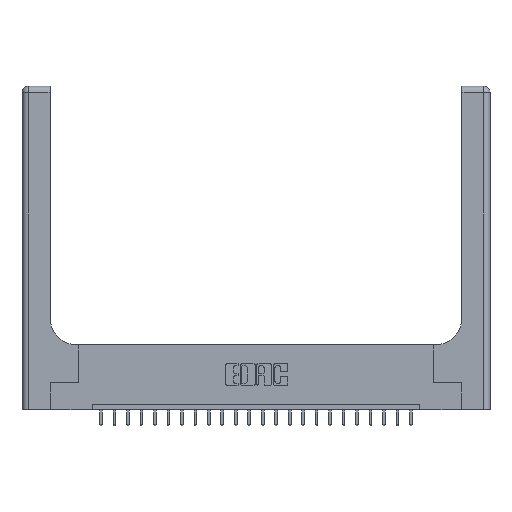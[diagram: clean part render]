
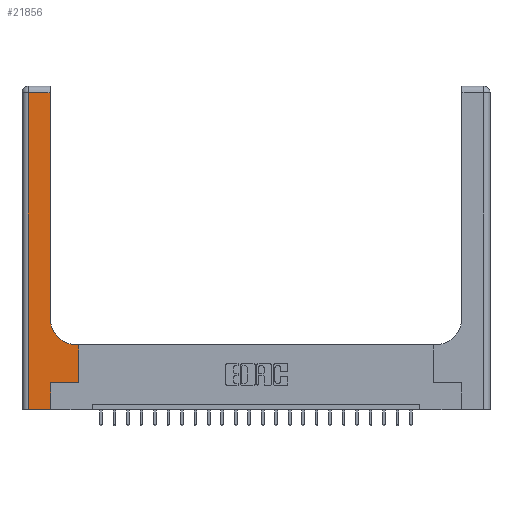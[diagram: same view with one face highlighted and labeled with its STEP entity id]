
A CAD part, top view. The second image highlights one B-rep face of the part: STEP entity #21856.
In plain terms, the highlighted planar face has unit normal (0, 0, 1).
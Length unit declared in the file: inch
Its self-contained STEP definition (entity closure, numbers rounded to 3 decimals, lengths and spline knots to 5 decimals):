
#232 = CARTESIAN_POINT ( 'NONE',  ( 0.265, 0.25, 0.37 ) ) ;
#1228 = CARTESIAN_POINT ( 'NONE',  ( 0.51, 0.6, 0.37 ) ) ;
#2026 = CARTESIAN_POINT ( 'NONE',  ( 0.265, 0., 0.37 ) ) ;
#2142 = DIRECTION ( 'NONE',  ( -1., 0., 0. ) ) ;
#2154 = DIRECTION ( 'NONE',  ( 1., 0., 0. ) ) ;
#2218 = CARTESIAN_POINT ( 'NONE',  ( 0.06, 2.94, 0.37 ) ) ;
#2223 = CARTESIAN_POINT ( 'NONE',  ( 0., 0., 0.37 ) ) ;
#2245 = PLANE ( 'NONE',  #7970 ) ;
#2419 = CARTESIAN_POINT ( 'NONE',  ( 0.528, 0.25, 0.37 ) ) ;
#2725 = DIRECTION ( 'NONE',  ( -1., 0., 0. ) ) ;
#2864 = VERTEX_POINT ( 'NONE', #14669 ) ;
#3715 = CARTESIAN_POINT ( 'NONE',  ( 0.06, 0., 0.37 ) ) ;
#4055 = CARTESIAN_POINT ( 'NONE',  ( 0., 2.94, 0.37 ) ) ;
#4107 = DIRECTION ( 'NONE',  ( 0., 0., -1. ) ) ;
#4255 = VECTOR ( 'NONE', #16063, 39.37008 ) ;
#4325 = DIRECTION ( 'NONE',  ( 0., 0., -1. ) ) ;
#4984 = ORIENTED_EDGE ( 'NONE', *, *, #13553, .T. ) ;
#5240 = VECTOR ( 'NONE', #17815, 39.37008 ) ;
#6204 = LINE ( 'NONE', #20498, #13861 ) ;
#6230 = EDGE_LOOP ( 'NONE', ( #4984, #18419, #7827, #17557, #17902, #16923, #7605, #18739, #9390 ) ) ;
#6245 = LINE ( 'NONE', #2419, #9739 ) ;
#7581 = FACE_OUTER_BOUND ( 'NONE', #6230, .T. ) ;
#7605 = ORIENTED_EDGE ( 'NONE', *, *, #14408, .T. ) ;
#7763 = DIRECTION ( 'NONE',  ( -1., 0., 0. ) ) ;
#7827 = ORIENTED_EDGE ( 'NONE', *, *, #8521, .T. ) ;
#7970 = AXIS2_PLACEMENT_3D ( 'NONE', #19796, #4325, #2142 ) ;
#7999 = LINE ( 'NONE', #4055, #13458 ) ;
#8104 = DIRECTION ( 'NONE',  ( 0., 1., 0. ) ) ;
#8521 = EDGE_CURVE ( 'NONE', #12665, #9909, #20924, .T. ) ;
#8888 = VERTEX_POINT ( 'NONE', #20872 ) ;
#8959 = CARTESIAN_POINT ( 'NONE',  ( 0.26, 0.85, 0.37 ) ) ;
#8989 = LINE ( 'NONE', #2026, #4255 ) ;
#9312 = VECTOR ( 'NONE', #18268, 39.37008 ) ;
#9390 = ORIENTED_EDGE ( 'NONE', *, *, #18151, .T. ) ;
#9608 = VERTEX_POINT ( 'NONE', #11747 ) ;
#9717 = VECTOR ( 'NONE', #21618, 39.37008 ) ;
#9739 = VECTOR ( 'NONE', #8104, 39.37008 ) ;
#9909 = VERTEX_POINT ( 'NONE', #3715 ) ;
#10444 = AXIS2_PLACEMENT_3D ( 'NONE', #21772, #4107, #2154 ) ;
#10702 = VECTOR ( 'NONE', #14161, 39.37008 ) ;
#11173 = LINE ( 'NONE', #18052, #9312 ) ;
#11747 = CARTESIAN_POINT ( 'NONE',  ( 0.528, 0.25, 0.37 ) ) ;
#12427 = CARTESIAN_POINT ( 'NONE',  ( 0.06, 3., 0.37 ) ) ;
#12665 = VERTEX_POINT ( 'NONE', #2218 ) ;
#12693 = CARTESIAN_POINT ( 'NONE',  ( 0.26, 3., 0.37 ) ) ;
#13458 = VECTOR ( 'NONE', #7763, 39.37008 ) ;
#13553 = EDGE_CURVE ( 'NONE', #13951, #2864, #19564, .T. ) ;
#13580 = EDGE_CURVE ( 'NONE', #14258, #9608, #11173, .T. ) ;
#13861 = VECTOR ( 'NONE', #2725, 39.37008 ) ;
#13922 = EDGE_CURVE ( 'NONE', #9909, #8888, #14291, .T. ) ;
#13951 = VERTEX_POINT ( 'NONE', #8959 ) ;
#14161 = DIRECTION ( 'NONE',  ( 0., -1., 0. ) ) ;
#14258 = VERTEX_POINT ( 'NONE', #232 ) ;
#14291 = LINE ( 'NONE', #2223, #9717 ) ;
#14408 = EDGE_CURVE ( 'NONE', #9608, #15280, #6245, .T. ) ;
#14669 = CARTESIAN_POINT ( 'NONE',  ( 0.26, 2.94, 0.37 ) ) ;
#15280 = VERTEX_POINT ( 'NONE', #17758 ) ;
#16063 = DIRECTION ( 'NONE',  ( 0., 1., 0. ) ) ;
#16923 = ORIENTED_EDGE ( 'NONE', *, *, #13580, .T. ) ;
#17557 = ORIENTED_EDGE ( 'NONE', *, *, #13922, .T. ) ;
#17758 = CARTESIAN_POINT ( 'NONE',  ( 0.528, 0.6, 0.37 ) ) ;
#17815 = DIRECTION ( 'NONE',  ( 0., 1., 0. ) ) ;
#17902 = ORIENTED_EDGE ( 'NONE', *, *, #21754, .T. ) ;
#18052 = CARTESIAN_POINT ( 'NONE',  ( 0.265, 0.25, 0.37 ) ) ;
#18151 = EDGE_CURVE ( 'NONE', #21519, #13951, #22324, .T. ) ;
#18268 = DIRECTION ( 'NONE',  ( 1., 0., 0. ) ) ;
#18419 = ORIENTED_EDGE ( 'NONE', *, *, #19125, .T. ) ;
#18739 = ORIENTED_EDGE ( 'NONE', *, *, #20160, .T. ) ;
#19125 = EDGE_CURVE ( 'NONE', #2864, #12665, #7999, .T. ) ;
#19564 = LINE ( 'NONE', #12693, #5240 ) ;
#19796 = CARTESIAN_POINT ( 'NONE',  ( 0., 3., 0.37 ) ) ;
#20160 = EDGE_CURVE ( 'NONE', #15280, #21519, #6204, .T. ) ;
#20498 = CARTESIAN_POINT ( 'NONE',  ( 0.26, 0.6, 0.37 ) ) ;
#20872 = CARTESIAN_POINT ( 'NONE',  ( 0.265, 0., 0.37 ) ) ;
#20924 = LINE ( 'NONE', #12427, #10702 ) ;
#21519 = VERTEX_POINT ( 'NONE', #1228 ) ;
#21618 = DIRECTION ( 'NONE',  ( 1., 0., 0. ) ) ;
#21754 = EDGE_CURVE ( 'NONE', #8888, #14258, #8989, .T. ) ;
#21772 = CARTESIAN_POINT ( 'NONE',  ( 0.51, 0.85, 0.37 ) ) ;
#21856 = ADVANCED_FACE ( 'NONE', ( #7581 ), #2245, .F. ) ;
#22324 = CIRCLE ( 'NONE', #10444, 0.25 ) ;
